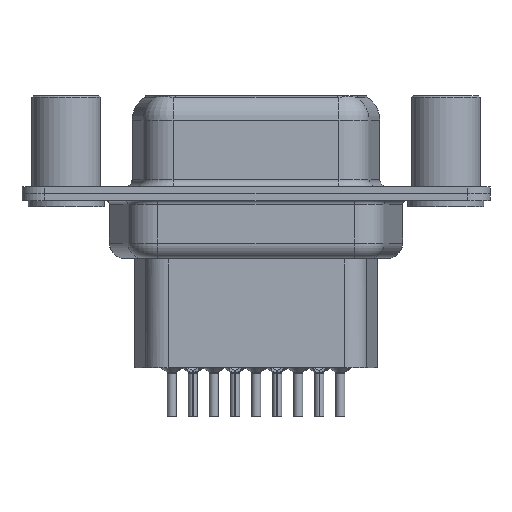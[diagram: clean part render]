
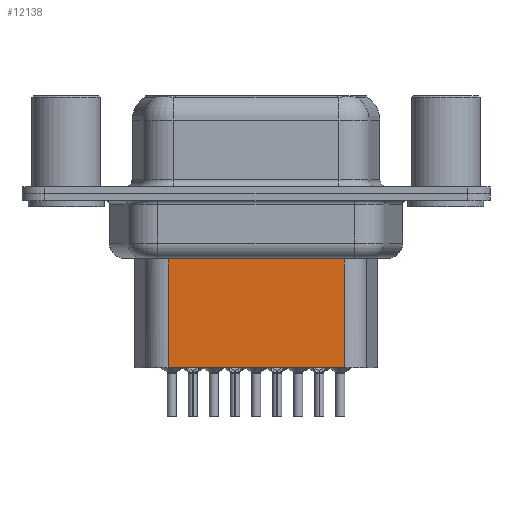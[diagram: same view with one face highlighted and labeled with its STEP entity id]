
A CAD part, front view. The second image highlights one B-rep face of the part: STEP entity #12138.
In plain terms, the highlighted planar face has unit normal (0, -1, 0).
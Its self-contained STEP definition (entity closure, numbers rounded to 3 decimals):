
#981 = CARTESIAN_POINT ( 'NONE',  ( 18.294, -3.5, -11.45 ) ) ;
#1585 = EDGE_CURVE ( 'NONE', #2023, #18185, #14354, .T. ) ;
#2023 = VERTEX_POINT ( 'NONE', #7169 ) ;
#2214 = DIRECTION ( 'NONE',  ( 0., 0., -1. ) ) ;
#3877 = VERTEX_POINT ( 'NONE', #3898 ) ;
#3898 = CARTESIAN_POINT ( 'NONE',  ( 18.294, -3.5, -4.097 ) ) ;
#4389 = CARTESIAN_POINT ( 'NONE',  ( 6.706, -3.5, -11.45 ) ) ;
#4397 = AXIS2_PLACEMENT_3D ( 'NONE', #5485, #19418, #9007 ) ;
#5175 = VECTOR ( 'NONE', #2214, 1000. ) ;
#5485 = CARTESIAN_POINT ( 'NONE',  ( 6.706, -3.5, -3.1 ) ) ;
#7169 = CARTESIAN_POINT ( 'NONE',  ( 6.706, -3.5, -4.097 ) ) ;
#7196 = PLANE ( 'NONE',  #4397 ) ;
#7610 = VECTOR ( 'NONE', #20730, 1000. ) ;
#8054 = VECTOR ( 'NONE', #16923, 1000. ) ;
#8163 = LINE ( 'NONE', #10326, #7610 ) ;
#8181 = LINE ( 'NONE', #4389, #12793 ) ;
#8452 = ORIENTED_EDGE ( 'NONE', *, *, #11900, .F. ) ;
#8862 = FACE_OUTER_BOUND ( 'NONE', #9298, .T. ) ;
#9007 = DIRECTION ( 'NONE',  ( 1., 0., 0. ) ) ;
#9085 = ORIENTED_EDGE ( 'NONE', *, *, #1585, .T. ) ;
#9298 = EDGE_LOOP ( 'NONE', ( #8452, #10728, #9085, #11514 ) ) ;
#9920 = CARTESIAN_POINT ( 'NONE',  ( 18.294, -3.5, -3.1 ) ) ;
#10326 = CARTESIAN_POINT ( 'NONE',  ( 6.459, -3.5, -4.097 ) ) ;
#10728 = ORIENTED_EDGE ( 'NONE', *, *, #19356, .T. ) ;
#11514 = ORIENTED_EDGE ( 'NONE', *, *, #17690, .F. ) ;
#11900 = EDGE_CURVE ( 'NONE', #3877, #12556, #13220, .T. ) ;
#12138 = ADVANCED_FACE ( 'NONE', ( #8862 ), #7196, .T. ) ;
#12556 = VERTEX_POINT ( 'NONE', #981 ) ;
#12793 = VECTOR ( 'NONE', #14752, 1000. ) ;
#13220 = LINE ( 'NONE', #9920, #8054 ) ;
#14354 = LINE ( 'NONE', #15981, #5175 ) ;
#14752 = DIRECTION ( 'NONE',  ( -1., 0., 0. ) ) ;
#15981 = CARTESIAN_POINT ( 'NONE',  ( 6.706, -3.5, -3.1 ) ) ;
#16923 = DIRECTION ( 'NONE',  ( 0., 0., -1. ) ) ;
#17690 = EDGE_CURVE ( 'NONE', #12556, #18185, #8181, .T. ) ;
#17850 = CARTESIAN_POINT ( 'NONE',  ( 6.706, -3.5, -11.45 ) ) ;
#18185 = VERTEX_POINT ( 'NONE', #17850 ) ;
#19356 = EDGE_CURVE ( 'NONE', #3877, #2023, #8163, .T. ) ;
#19418 = DIRECTION ( 'NONE',  ( 0., -1., 0. ) ) ;
#20730 = DIRECTION ( 'NONE',  ( -1., 0., 0. ) ) ;
